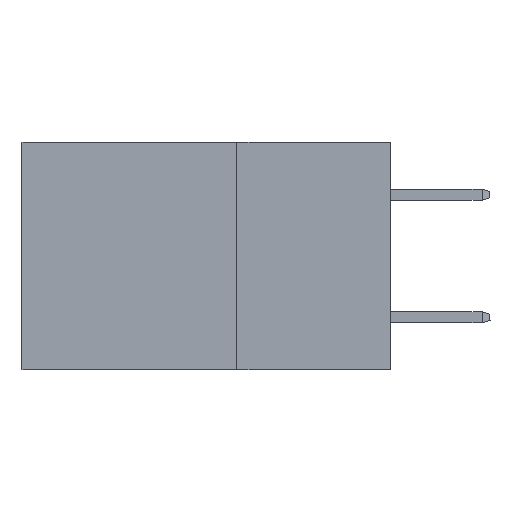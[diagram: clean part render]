
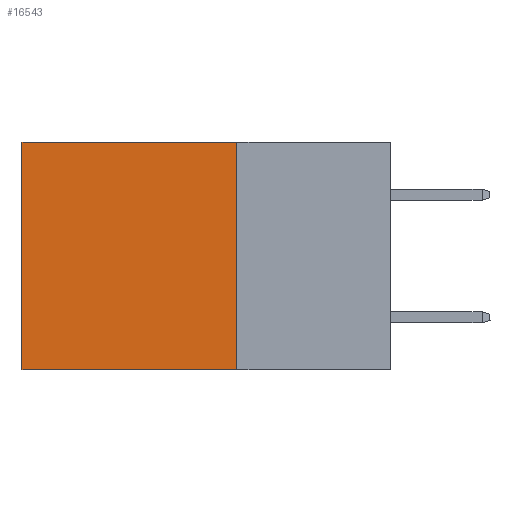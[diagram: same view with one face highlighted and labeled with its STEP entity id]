
A CAD part, left-side view. The second image highlights one B-rep face of the part: STEP entity #16543.
In plain terms, the highlighted planar face has unit normal (-1, 0, 0).
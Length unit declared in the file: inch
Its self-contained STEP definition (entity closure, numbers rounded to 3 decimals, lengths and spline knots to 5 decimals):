
#11 = CARTESIAN_POINT ( 'NONE',  ( 0.2875, 0.25, 0. ) ) ;
#853 = LINE ( 'NONE', #9992, #17438 ) ;
#1004 = DIRECTION ( 'NONE',  ( 0., 0., -1. ) ) ;
#1201 = VECTOR ( 'NONE', #17075, 39.37008 ) ;
#1667 = CARTESIAN_POINT ( 'NONE',  ( 0.2875, 0.6, -0.37 ) ) ;
#1954 = DIRECTION ( 'NONE',  ( 0., 1., 0. ) ) ;
#2256 = VERTEX_POINT ( 'NONE', #11 ) ;
#2668 = VECTOR ( 'NONE', #1954, 39.37008 ) ;
#4357 = ORIENTED_EDGE ( 'NONE', *, *, #6519, .F. ) ;
#4813 = DIRECTION ( 'NONE',  ( 1., 0., 0. ) ) ;
#6307 = EDGE_CURVE ( 'NONE', #12927, #10849, #14023, .T. ) ;
#6316 = CARTESIAN_POINT ( 'NONE',  ( 0.2875, 0.25, 0. ) ) ;
#6404 = VECTOR ( 'NONE', #1004, 39.37008 ) ;
#6430 = AXIS2_PLACEMENT_3D ( 'NONE', #17069, #4813, #10869 ) ;
#6519 = EDGE_CURVE ( 'NONE', #2256, #12927, #853, .T. ) ;
#6951 = DIRECTION ( 'NONE',  ( 0., 0., -1. ) ) ;
#7820 = PLANE ( 'NONE',  #6430 ) ;
#9743 = ORIENTED_EDGE ( 'NONE', *, *, #15659, .T. ) ;
#9992 = CARTESIAN_POINT ( 'NONE',  ( 0.2875, 0.25, 0. ) ) ;
#10849 = VERTEX_POINT ( 'NONE', #1667 ) ;
#10869 = DIRECTION ( 'NONE',  ( 0., 0., -1. ) ) ;
#11043 = CARTESIAN_POINT ( 'NONE',  ( 0.2875, 0.25, -0.37 ) ) ;
#11477 = EDGE_LOOP ( 'NONE', ( #9743, #13378, #4357, #15614 ) ) ;
#12927 = VERTEX_POINT ( 'NONE', #11043 ) ;
#13378 = ORIENTED_EDGE ( 'NONE', *, *, #6307, .F. ) ;
#13462 = LINE ( 'NONE', #15161, #6404 ) ;
#14023 = LINE ( 'NONE', #15735, #2668 ) ;
#15161 = CARTESIAN_POINT ( 'NONE',  ( 0.2875, 0.6, 0. ) ) ;
#15614 = ORIENTED_EDGE ( 'NONE', *, *, #18324, .T. ) ;
#15659 = EDGE_CURVE ( 'NONE', #16763, #10849, #13462, .T. ) ;
#15735 = CARTESIAN_POINT ( 'NONE',  ( 0.2875, 0.25, -0.37 ) ) ;
#16543 = ADVANCED_FACE ( 'NONE', ( #17269 ), #7820, .F. ) ;
#16693 = LINE ( 'NONE', #6316, #1201 ) ;
#16763 = VERTEX_POINT ( 'NONE', #17650 ) ;
#17069 = CARTESIAN_POINT ( 'NONE',  ( 0.2875, 0.25, 0. ) ) ;
#17075 = DIRECTION ( 'NONE',  ( 0., 1., 0. ) ) ;
#17269 = FACE_OUTER_BOUND ( 'NONE', #11477, .T. ) ;
#17438 = VECTOR ( 'NONE', #6951, 39.37008 ) ;
#17650 = CARTESIAN_POINT ( 'NONE',  ( 0.2875, 0.6, 0. ) ) ;
#18324 = EDGE_CURVE ( 'NONE', #2256, #16763, #16693, .T. ) ;
